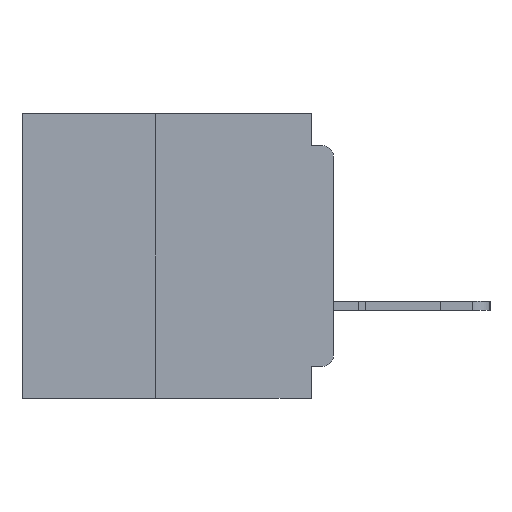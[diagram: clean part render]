
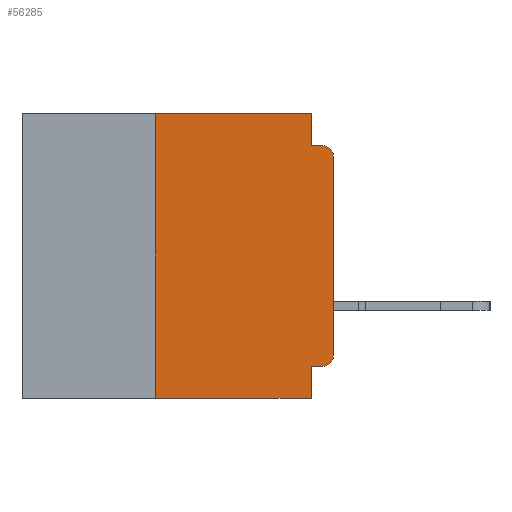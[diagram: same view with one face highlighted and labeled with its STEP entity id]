
A CAD part, left-side view. The second image highlights one B-rep face of the part: STEP entity #56285.
In plain terms, the highlighted planar face has unit normal (-1, 0, 0).
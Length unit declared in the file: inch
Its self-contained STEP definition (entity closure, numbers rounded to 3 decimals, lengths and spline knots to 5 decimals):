
#3298 = CARTESIAN_POINT ( 'NONE',  ( 0., 0., -0.355 ) ) ;
#4323 = VERTEX_POINT ( 'NONE', #8626 ) ;
#4607 = DIRECTION ( 'NONE',  ( -1., 0., 0. ) ) ;
#6860 = VECTOR ( 'NONE', #48118, 39.37008 ) ;
#6938 = ORIENTED_EDGE ( 'NONE', *, *, #58032, .T. ) ;
#7251 = ORIENTED_EDGE ( 'NONE', *, *, #12712, .F. ) ;
#8626 = CARTESIAN_POINT ( 'NONE',  ( 0., 0.031, -0.045 ) ) ;
#8927 = EDGE_CURVE ( 'NONE', #28047, #19052, #61108, .T. ) ;
#9258 = CARTESIAN_POINT ( 'NONE',  ( 0., 0.031, 0. ) ) ;
#9371 = AXIS2_PLACEMENT_3D ( 'NONE', #55229, #26174, #60108 ) ;
#9615 = ORIENTED_EDGE ( 'NONE', *, *, #43567, .F. ) ;
#10050 = EDGE_CURVE ( 'NONE', #13474, #26280, #23859, .T. ) ;
#11967 = DIRECTION ( 'NONE',  ( 0., 0., 1. ) ) ;
#12712 = EDGE_CURVE ( 'NONE', #51113, #42172, #20594, .T. ) ;
#13474 = VERTEX_POINT ( 'NONE', #53429 ) ;
#14085 = CARTESIAN_POINT ( 'NONE',  ( 0., 0.437, -0.4 ) ) ;
#16110 = CARTESIAN_POINT ( 'NONE',  ( 0., 0.015, -0.34 ) ) ;
#17162 = LINE ( 'NONE', #59305, #30167 ) ;
#18431 = AXIS2_PLACEMENT_3D ( 'NONE', #33840, #4607, #38680 ) ;
#19052 = VERTEX_POINT ( 'NONE', #23391 ) ;
#19174 = CARTESIAN_POINT ( 'NONE',  ( 0., 0.015, -0.355 ) ) ;
#20079 = LINE ( 'NONE', #34701, #60333 ) ;
#20594 = LINE ( 'NONE', #3298, #43382 ) ;
#21019 = DIRECTION ( 'NONE',  ( 0., 0., -1. ) ) ;
#21880 = LINE ( 'NONE', #32009, #49259 ) ;
#22372 = LINE ( 'NONE', #44084, #35328 ) ;
#23391 = CARTESIAN_POINT ( 'NONE',  ( 0., 0.25, 0. ) ) ;
#23859 = LINE ( 'NONE', #51112, #25372 ) ;
#24685 = EDGE_CURVE ( 'NONE', #28047, #28622, #45706, .T. ) ;
#25336 = DIRECTION ( 'NONE',  ( 0., -1., 0. ) ) ;
#25372 = VECTOR ( 'NONE', #11967, 39.37008 ) ;
#26015 = ORIENTED_EDGE ( 'NONE', *, *, #62932, .F. ) ;
#26174 = DIRECTION ( 'NONE',  ( 1., 0., 0. ) ) ;
#26280 = VERTEX_POINT ( 'NONE', #46644 ) ;
#27283 = EDGE_LOOP ( 'NONE', ( #51030, #6938, #48767, #36347, #26015, #48126, #54341, #9615, #7251, #28433 ) ) ;
#28047 = VERTEX_POINT ( 'NONE', #34108 ) ;
#28433 = ORIENTED_EDGE ( 'NONE', *, *, #33428, .T. ) ;
#28622 = VERTEX_POINT ( 'NONE', #43125 ) ;
#29222 = AXIS2_PLACEMENT_3D ( 'NONE', #16110, #50123, #21019 ) ;
#30167 = VECTOR ( 'NONE', #25336, 39.37008 ) ;
#32009 = CARTESIAN_POINT ( 'NONE',  ( 0., 0.031, -0.4 ) ) ;
#32471 = CIRCLE ( 'NONE', #29222, 0.015 ) ;
#32536 = DIRECTION ( 'NONE',  ( 0., 1., 0. ) ) ;
#33428 = EDGE_CURVE ( 'NONE', #51113, #13474, #32471, .T. ) ;
#33840 = CARTESIAN_POINT ( 'NONE',  ( 0., 0.015, -0.06 ) ) ;
#34108 = CARTESIAN_POINT ( 'NONE',  ( 0., 0.25, -0.4 ) ) ;
#34701 = CARTESIAN_POINT ( 'NONE',  ( 0., 0.437, 0. ) ) ;
#35328 = VECTOR ( 'NONE', #48971, 39.37008 ) ;
#36347 = ORIENTED_EDGE ( 'NONE', *, *, #49307, .F. ) ;
#36659 = CARTESIAN_POINT ( 'NONE',  ( 0., 0.015, -0.045 ) ) ;
#36872 = DIRECTION ( 'NONE',  ( 0., 0., -1. ) ) ;
#38680 = DIRECTION ( 'NONE',  ( 0., 0., -1. ) ) ;
#40619 = PLANE ( 'NONE',  #9371 ) ;
#42172 = VERTEX_POINT ( 'NONE', #49547 ) ;
#43125 = CARTESIAN_POINT ( 'NONE',  ( 0., 0.031, -0.4 ) ) ;
#43382 = VECTOR ( 'NONE', #32536, 39.37008 ) ;
#43567 = EDGE_CURVE ( 'NONE', #42172, #28622, #21880, .T. ) ;
#44084 = CARTESIAN_POINT ( 'NONE',  ( 0., 0.031, 0. ) ) ;
#44795 = DIRECTION ( 'NONE',  ( 0., 0., 1. ) ) ;
#45706 = LINE ( 'NONE', #14085, #6860 ) ;
#45757 = VERTEX_POINT ( 'NONE', #36659 ) ;
#45832 = FACE_OUTER_BOUND ( 'NONE', #27283, .T. ) ;
#46644 = CARTESIAN_POINT ( 'NONE',  ( 0., 0., -0.06 ) ) ;
#48118 = DIRECTION ( 'NONE',  ( 0., -1., 0. ) ) ;
#48126 = ORIENTED_EDGE ( 'NONE', *, *, #8927, .F. ) ;
#48223 = VECTOR ( 'NONE', #44795, 39.37008 ) ;
#48658 = CIRCLE ( 'NONE', #18431, 0.015 ) ;
#48767 = ORIENTED_EDGE ( 'NONE', *, *, #61054, .F. ) ;
#48971 = DIRECTION ( 'NONE',  ( 0., 0., -1. ) ) ;
#49259 = VECTOR ( 'NONE', #36872, 39.37008 ) ;
#49307 = EDGE_CURVE ( 'NONE', #54583, #4323, #22372, .T. ) ;
#49482 = CARTESIAN_POINT ( 'NONE',  ( 0., 0.25, -0.4 ) ) ;
#49547 = CARTESIAN_POINT ( 'NONE',  ( 0., 0.031, -0.355 ) ) ;
#50123 = DIRECTION ( 'NONE',  ( -1., 0., 0. ) ) ;
#51030 = ORIENTED_EDGE ( 'NONE', *, *, #10050, .T. ) ;
#51112 = CARTESIAN_POINT ( 'NONE',  ( 0., 0., 0. ) ) ;
#51113 = VERTEX_POINT ( 'NONE', #19174 ) ;
#53429 = CARTESIAN_POINT ( 'NONE',  ( 0., 0., -0.34 ) ) ;
#53989 = DIRECTION ( 'NONE',  ( 0., -1., 0. ) ) ;
#54341 = ORIENTED_EDGE ( 'NONE', *, *, #24685, .T. ) ;
#54583 = VERTEX_POINT ( 'NONE', #9258 ) ;
#55229 = CARTESIAN_POINT ( 'NONE',  ( 0., 0.437, 0. ) ) ;
#56285 = ADVANCED_FACE ( 'NONE', ( #45832 ), #40619, .F. ) ;
#58032 = EDGE_CURVE ( 'NONE', #26280, #45757, #48658, .T. ) ;
#59305 = CARTESIAN_POINT ( 'NONE',  ( 0., 0., -0.045 ) ) ;
#60108 = DIRECTION ( 'NONE',  ( 0., 0., -1. ) ) ;
#60333 = VECTOR ( 'NONE', #53989, 39.37008 ) ;
#61054 = EDGE_CURVE ( 'NONE', #4323, #45757, #17162, .T. ) ;
#61108 = LINE ( 'NONE', #49482, #48223 ) ;
#62932 = EDGE_CURVE ( 'NONE', #19052, #54583, #20079, .T. ) ;
